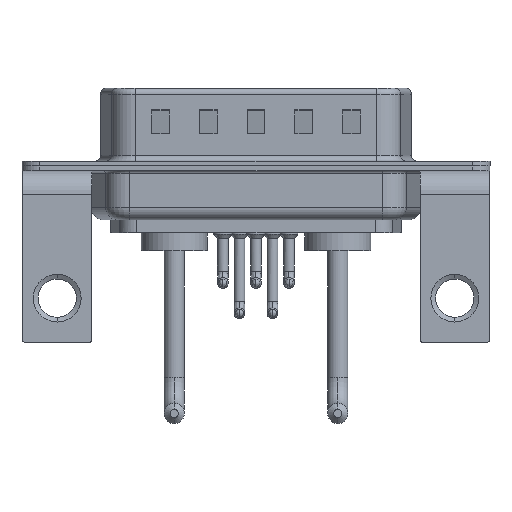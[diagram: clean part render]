
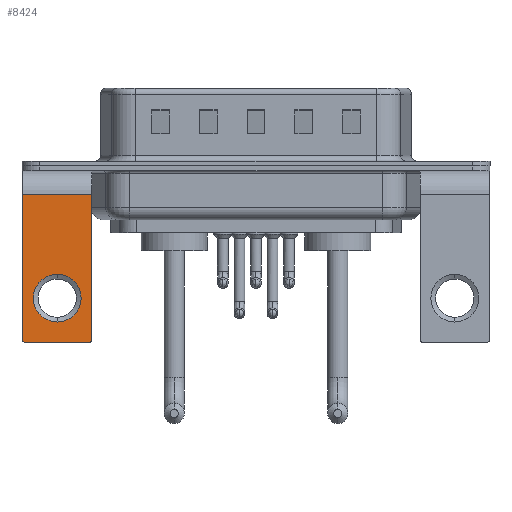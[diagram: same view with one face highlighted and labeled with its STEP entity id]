
A CAD part, front view. The second image highlights one B-rep face of the part: STEP entity #8424.
In plain terms, the highlighted planar face has unit normal (0, -1, 0).
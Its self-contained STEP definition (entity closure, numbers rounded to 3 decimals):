
#285 = CARTESIAN_POINT ( 'NONE',  ( 2.65, -6.25, -14.55 ) ) ;
#430 = VECTOR ( 'NONE', #15958, 1000. ) ;
#836 = FACE_BOUND ( 'NONE', #5712, .T. ) ;
#929 = LINE ( 'NONE', #12219, #11213 ) ;
#1379 = CARTESIAN_POINT ( 'NONE',  ( 0., -6.25, -11.07 ) ) ;
#1400 = VECTOR ( 'NONE', #7978, 1000. ) ;
#1677 = CARTESIAN_POINT ( 'NONE',  ( -2.9, -6.25, -2.4 ) ) ;
#1685 = CARTESIAN_POINT ( 'NONE',  ( -2.65, -6.25, -14.8 ) ) ;
#1783 = ORIENTED_EDGE ( 'NONE', *, *, #9793, .T. ) ;
#1940 = DIRECTION ( 'NONE',  ( 0., 0., 1. ) ) ;
#1966 = ORIENTED_EDGE ( 'NONE', *, *, #4852, .T. ) ;
#1979 = DIRECTION ( 'NONE',  ( 0., 0., 1. ) ) ;
#2096 = EDGE_CURVE ( 'NONE', #4494, #7755, #4159, .T. ) ;
#2198 = CARTESIAN_POINT ( 'NONE',  ( 0., -6.25, -13.07 ) ) ;
#2497 = EDGE_LOOP ( 'NONE', ( #4858, #15337, #9930, #14726, #5336, #1966 ) ) ;
#2722 = CARTESIAN_POINT ( 'NONE',  ( 0., -6.25, -9.07 ) ) ;
#2825 = DIRECTION ( 'NONE',  ( 0., 1., 0. ) ) ;
#3705 = CARTESIAN_POINT ( 'NONE',  ( 2.9, -6.25, -14.8 ) ) ;
#3802 = DIRECTION ( 'NONE',  ( 0., -1., 0. ) ) ;
#4159 = CIRCLE ( 'NONE', #16408, 2. ) ;
#4409 = EDGE_CURVE ( 'NONE', #21382, #16705, #18992, .T. ) ;
#4494 = VERTEX_POINT ( 'NONE', #2722 ) ;
#4852 = EDGE_CURVE ( 'NONE', #13885, #7259, #17293, .T. ) ;
#4858 = ORIENTED_EDGE ( 'NONE', *, *, #9736, .T. ) ;
#5148 = CARTESIAN_POINT ( 'NONE',  ( 2.9, -6.25, -2.4 ) ) ;
#5336 = ORIENTED_EDGE ( 'NONE', *, *, #10063, .F. ) ;
#5712 = EDGE_LOOP ( 'NONE', ( #1783, #13421 ) ) ;
#5800 = FACE_OUTER_BOUND ( 'NONE', #2497, .T. ) ;
#5917 = DIRECTION ( 'NONE',  ( 0., 1., 0. ) ) ;
#6125 = CARTESIAN_POINT ( 'NONE',  ( -2.65, -6.25, -14.55 ) ) ;
#6678 = AXIS2_PLACEMENT_3D ( 'NONE', #1379, #2825, #11146 ) ;
#7259 = VERTEX_POINT ( 'NONE', #1677 ) ;
#7545 = PLANE ( 'NONE',  #10659 ) ;
#7604 = VERTEX_POINT ( 'NONE', #16357 ) ;
#7755 = VERTEX_POINT ( 'NONE', #2198 ) ;
#7978 = DIRECTION ( 'NONE',  ( 0., 0., -1. ) ) ;
#8067 = DIRECTION ( 'NONE',  ( 0., 0., 1. ) ) ;
#8424 = ADVANCED_FACE ( 'NONE', ( #836, #5800 ), #7545, .F. ) ;
#9181 = AXIS2_PLACEMENT_3D ( 'NONE', #6125, #20534, #1979 ) ;
#9736 = EDGE_CURVE ( 'NONE', #7259, #21382, #16527, .T. ) ;
#9793 = EDGE_CURVE ( 'NONE', #7755, #4494, #17194, .T. ) ;
#9902 = CARTESIAN_POINT ( 'NONE',  ( -2.9, -6.25, -14.55 ) ) ;
#9930 = ORIENTED_EDGE ( 'NONE', *, *, #21170, .F. ) ;
#10063 = EDGE_CURVE ( 'NONE', #13885, #12211, #929, .T. ) ;
#10659 = AXIS2_PLACEMENT_3D ( 'NONE', #14220, #14877, #8067 ) ;
#10732 = CARTESIAN_POINT ( 'NONE',  ( 0., -6.25, -11.07 ) ) ;
#11146 = DIRECTION ( 'NONE',  ( 0., 0., 1. ) ) ;
#11213 = VECTOR ( 'NONE', #15852, 1000. ) ;
#11799 = LINE ( 'NONE', #3705, #20166 ) ;
#12211 = VERTEX_POINT ( 'NONE', #18659 ) ;
#12219 = CARTESIAN_POINT ( 'NONE',  ( 2.9, -6.25, -2.4 ) ) ;
#12540 = CARTESIAN_POINT ( 'NONE',  ( 2.9, -6.25, -2.4 ) ) ;
#13321 = CARTESIAN_POINT ( 'NONE',  ( -2.9, -6.25, -2.4 ) ) ;
#13421 = ORIENTED_EDGE ( 'NONE', *, *, #2096, .T. ) ;
#13885 = VERTEX_POINT ( 'NONE', #5148 ) ;
#14220 = CARTESIAN_POINT ( 'NONE',  ( 2.9, -6.25, -2.4 ) ) ;
#14339 = DIRECTION ( 'NONE',  ( 0., 0., 1. ) ) ;
#14726 = ORIENTED_EDGE ( 'NONE', *, *, #18974, .T. ) ;
#14877 = DIRECTION ( 'NONE',  ( 0., 1., 0. ) ) ;
#15337 = ORIENTED_EDGE ( 'NONE', *, *, #4409, .T. ) ;
#15852 = DIRECTION ( 'NONE',  ( 0., 0., -1. ) ) ;
#15958 = DIRECTION ( 'NONE',  ( -1., 0., 0. ) ) ;
#16357 = CARTESIAN_POINT ( 'NONE',  ( 2.65, -6.25, -14.8 ) ) ;
#16408 = AXIS2_PLACEMENT_3D ( 'NONE', #10732, #5917, #14339 ) ;
#16527 = LINE ( 'NONE', #13321, #1400 ) ;
#16705 = VERTEX_POINT ( 'NONE', #1685 ) ;
#17090 = DIRECTION ( 'NONE',  ( -1., 0., 0. ) ) ;
#17194 = CIRCLE ( 'NONE', #6678, 2. ) ;
#17293 = LINE ( 'NONE', #12540, #430 ) ;
#18399 = CIRCLE ( 'NONE', #21187, 0.25 ) ;
#18659 = CARTESIAN_POINT ( 'NONE',  ( 2.9, -6.25, -14.55 ) ) ;
#18974 = EDGE_CURVE ( 'NONE', #7604, #12211, #18399, .T. ) ;
#18992 = CIRCLE ( 'NONE', #9181, 0.25 ) ;
#20166 = VECTOR ( 'NONE', #17090, 1000. ) ;
#20534 = DIRECTION ( 'NONE',  ( 0., -1., 0. ) ) ;
#21170 = EDGE_CURVE ( 'NONE', #7604, #16705, #11799, .T. ) ;
#21187 = AXIS2_PLACEMENT_3D ( 'NONE', #285, #3802, #1940 ) ;
#21382 = VERTEX_POINT ( 'NONE', #9902 ) ;
